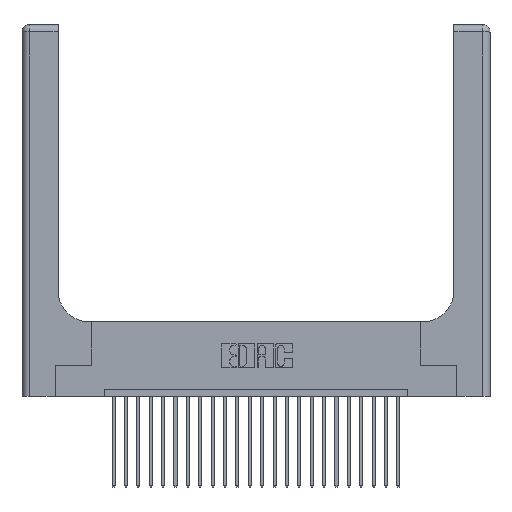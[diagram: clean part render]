
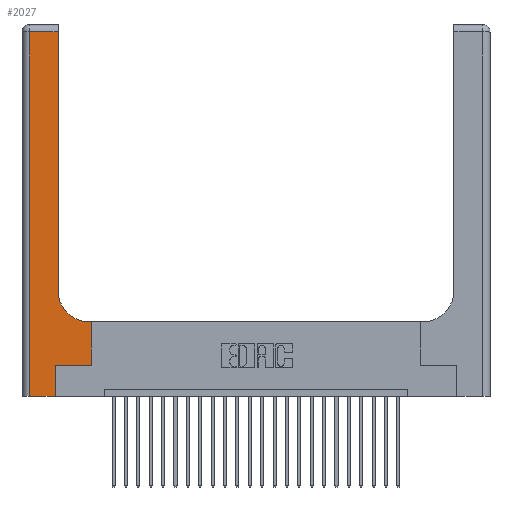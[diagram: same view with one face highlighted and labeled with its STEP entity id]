
A CAD part, top view. The second image highlights one B-rep face of the part: STEP entity #2027.
In plain terms, the highlighted planar face has unit normal (0, 0, 1).
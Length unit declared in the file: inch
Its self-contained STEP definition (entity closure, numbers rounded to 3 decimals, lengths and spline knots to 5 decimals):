
#38 = FACE_OUTER_BOUND ( 'NONE', #18597, .T. ) ;
#271 = DIRECTION ( 'NONE',  ( 1., 0., 0. ) ) ;
#546 = ORIENTED_EDGE ( 'NONE', *, *, #22013, .T. ) ;
#1157 = VECTOR ( 'NONE', #2155, 39.37008 ) ;
#1275 = EDGE_CURVE ( 'NONE', #6895, #21085, #2547, .T. ) ;
#1466 = LINE ( 'NONE', #7017, #24114 ) ;
#2027 = ADVANCED_FACE ( 'NONE', ( #38 ), #14544, .F. ) ;
#2155 = DIRECTION ( 'NONE',  ( 0., -1., 0. ) ) ;
#2547 = LINE ( 'NONE', #6323, #7814 ) ;
#3115 = ORIENTED_EDGE ( 'NONE', *, *, #6195, .T. ) ;
#3215 = LINE ( 'NONE', #13000, #13528 ) ;
#4239 = CARTESIAN_POINT ( 'NONE',  ( 0.5415, 0.85, 0.37 ) ) ;
#4384 = LINE ( 'NONE', #19347, #19280 ) ;
#4564 = AXIS2_PLACEMENT_3D ( 'NONE', #4239, #10365, #271 ) ;
#4944 = EDGE_CURVE ( 'NONE', #14541, #5709, #22848, .T. ) ;
#5556 = CARTESIAN_POINT ( 'NONE',  ( 0.269, 0., 0.37 ) ) ;
#5709 = VERTEX_POINT ( 'NONE', #12310 ) ;
#5829 = VERTEX_POINT ( 'NONE', #22593 ) ;
#6195 = EDGE_CURVE ( 'NONE', #12756, #5829, #3215, .T. ) ;
#6236 = DIRECTION ( 'NONE',  ( -1., 0., 0. ) ) ;
#6323 = CARTESIAN_POINT ( 'NONE',  ( 0.269, 0., 0.37 ) ) ;
#6895 = VERTEX_POINT ( 'NONE', #5556 ) ;
#7017 = CARTESIAN_POINT ( 'NONE',  ( 0., 2.94, 0.37 ) ) ;
#7198 = VERTEX_POINT ( 'NONE', #18500 ) ;
#7209 = ORIENTED_EDGE ( 'NONE', *, *, #7605, .T. ) ;
#7605 = EDGE_CURVE ( 'NONE', #5829, #13072, #25549, .T. ) ;
#7814 = VECTOR ( 'NONE', #24895, 39.37008 ) ;
#8097 = DIRECTION ( 'NONE',  ( 1., 0., 0. ) ) ;
#8904 = EDGE_CURVE ( 'NONE', #10824, #12756, #4384, .T. ) ;
#9443 = EDGE_CURVE ( 'NONE', #13072, #7198, #14947, .T. ) ;
#10365 = DIRECTION ( 'NONE',  ( 0., 0., -1. ) ) ;
#10468 = ORIENTED_EDGE ( 'NONE', *, *, #8904, .T. ) ;
#10681 = ORIENTED_EDGE ( 'NONE', *, *, #9443, .T. ) ;
#10783 = DIRECTION ( 'NONE',  ( 1., 0., 0. ) ) ;
#10824 = VERTEX_POINT ( 'NONE', #13148 ) ;
#11324 = DIRECTION ( 'NONE',  ( 0., 1., 0. ) ) ;
#12310 = CARTESIAN_POINT ( 'NONE',  ( 0.06, 0., 0.37 ) ) ;
#12756 = VERTEX_POINT ( 'NONE', #21868 ) ;
#12787 = VECTOR ( 'NONE', #22295, 39.37008 ) ;
#13000 = CARTESIAN_POINT ( 'NONE',  ( 0.2915, 0.6, 0.37 ) ) ;
#13072 = VERTEX_POINT ( 'NONE', #13124 ) ;
#13124 = CARTESIAN_POINT ( 'NONE',  ( 0.2915, 0.85, 0.37 ) ) ;
#13148 = CARTESIAN_POINT ( 'NONE',  ( 0.5585, 0.25, 0.37 ) ) ;
#13528 = VECTOR ( 'NONE', #14993, 39.37008 ) ;
#13798 = ORIENTED_EDGE ( 'NONE', *, *, #1275, .T. ) ;
#13846 = CARTESIAN_POINT ( 'NONE',  ( 0., 0., 0.37 ) ) ;
#14541 = VERTEX_POINT ( 'NONE', #18743 ) ;
#14544 = PLANE ( 'NONE',  #16518 ) ;
#14947 = LINE ( 'NONE', #24295, #12787 ) ;
#14993 = DIRECTION ( 'NONE',  ( -1., 0., 0. ) ) ;
#15452 = ORIENTED_EDGE ( 'NONE', *, *, #4944, .T. ) ;
#16088 = LINE ( 'NONE', #18903, #18577 ) ;
#16172 = ORIENTED_EDGE ( 'NONE', *, *, #16617, .T. ) ;
#16426 = EDGE_CURVE ( 'NONE', #7198, #14541, #1466, .T. ) ;
#16518 = AXIS2_PLACEMENT_3D ( 'NONE', #20587, #21955, #6236 ) ;
#16617 = EDGE_CURVE ( 'NONE', #5709, #6895, #18862, .T. ) ;
#18500 = CARTESIAN_POINT ( 'NONE',  ( 0.2915, 2.94, 0.37 ) ) ;
#18577 = VECTOR ( 'NONE', #10783, 39.37008 ) ;
#18597 = EDGE_LOOP ( 'NONE', ( #10681, #19257, #15452, #16172, #13798, #546, #10468, #3115, #7209 ) ) ;
#18743 = CARTESIAN_POINT ( 'NONE',  ( 0.06, 2.94, 0.37 ) ) ;
#18862 = LINE ( 'NONE', #13846, #21332 ) ;
#18903 = CARTESIAN_POINT ( 'NONE',  ( 0.269, 0.25, 0.37 ) ) ;
#19257 = ORIENTED_EDGE ( 'NONE', *, *, #16426, .T. ) ;
#19280 = VECTOR ( 'NONE', #11324, 39.37008 ) ;
#19347 = CARTESIAN_POINT ( 'NONE',  ( 0.5585, 0.25, 0.37 ) ) ;
#20587 = CARTESIAN_POINT ( 'NONE',  ( 0., 3., 0.37 ) ) ;
#21085 = VERTEX_POINT ( 'NONE', #23405 ) ;
#21332 = VECTOR ( 'NONE', #8097, 39.37008 ) ;
#21868 = CARTESIAN_POINT ( 'NONE',  ( 0.5585, 0.6, 0.37 ) ) ;
#21955 = DIRECTION ( 'NONE',  ( 0., 0., -1. ) ) ;
#22013 = EDGE_CURVE ( 'NONE', #21085, #10824, #16088, .T. ) ;
#22295 = DIRECTION ( 'NONE',  ( 0., 1., 0. ) ) ;
#22593 = CARTESIAN_POINT ( 'NONE',  ( 0.5415, 0.6, 0.37 ) ) ;
#22848 = LINE ( 'NONE', #23141, #1157 ) ;
#22870 = DIRECTION ( 'NONE',  ( -1., 0., 0. ) ) ;
#23141 = CARTESIAN_POINT ( 'NONE',  ( 0.06, 3., 0.37 ) ) ;
#23405 = CARTESIAN_POINT ( 'NONE',  ( 0.269, 0.25, 0.37 ) ) ;
#24114 = VECTOR ( 'NONE', #22870, 39.37008 ) ;
#24295 = CARTESIAN_POINT ( 'NONE',  ( 0.2915, 3., 0.37 ) ) ;
#24895 = DIRECTION ( 'NONE',  ( 0., 1., 0. ) ) ;
#25549 = CIRCLE ( 'NONE', #4564, 0.25 ) ;
